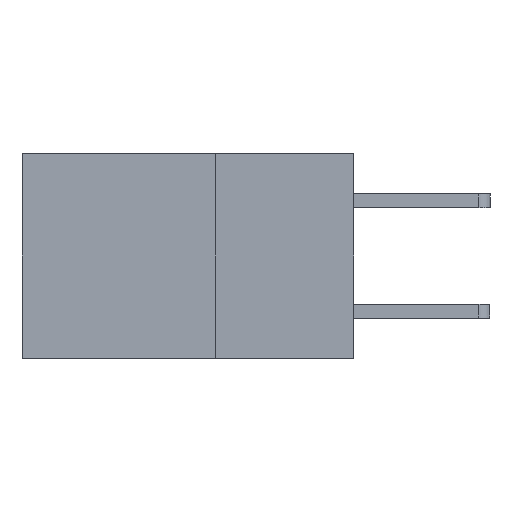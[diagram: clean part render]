
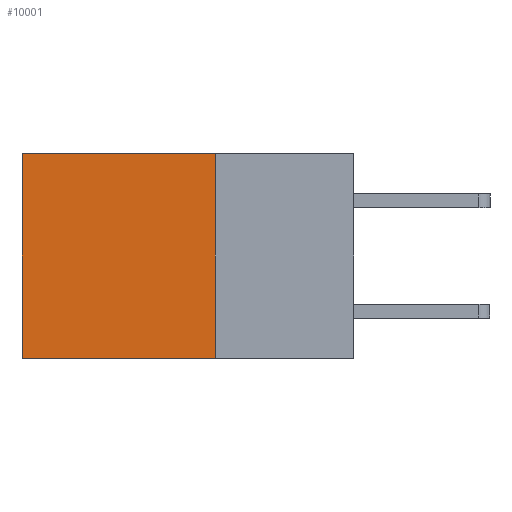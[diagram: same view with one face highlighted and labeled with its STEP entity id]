
A CAD part, left-side view. The second image highlights one B-rep face of the part: STEP entity #10001.
In plain terms, the highlighted planar face has unit normal (-1, 0, 0).
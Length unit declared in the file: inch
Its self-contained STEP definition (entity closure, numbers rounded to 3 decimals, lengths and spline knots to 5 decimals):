
#481 = CARTESIAN_POINT ( 'NONE',  ( 0.2875, 0.6, 0. ) ) ;
#626 = DIRECTION ( 'NONE',  ( 0., 0., -1. ) ) ;
#1221 = CARTESIAN_POINT ( 'NONE',  ( 0.2875, 0.25, 0. ) ) ;
#1279 = CARTESIAN_POINT ( 'NONE',  ( 0.2875, 0.25, 0. ) ) ;
#1508 = CARTESIAN_POINT ( 'NONE',  ( 0.2875, 0.6, -0.37 ) ) ;
#1657 = EDGE_CURVE ( 'NONE', #10789, #1830, #7637, .T. ) ;
#1830 = VERTEX_POINT ( 'NONE', #9324 ) ;
#2373 = EDGE_CURVE ( 'NONE', #10789, #7812, #5882, .T. ) ;
#2756 = EDGE_LOOP ( 'NONE', ( #9676, #6191, #10970, #8024 ) ) ;
#2924 = DIRECTION ( 'NONE',  ( 0., 0., -1. ) ) ;
#2990 = PLANE ( 'NONE',  #8286 ) ;
#3038 = DIRECTION ( 'NONE',  ( 1., 0., 0. ) ) ;
#3912 = VERTEX_POINT ( 'NONE', #1508 ) ;
#4685 = VECTOR ( 'NONE', #9892, 39.37008 ) ;
#5512 = DIRECTION ( 'NONE',  ( 0., 1., 0. ) ) ;
#5693 = DIRECTION ( 'NONE',  ( 0., 1., 0. ) ) ;
#5858 = CARTESIAN_POINT ( 'NONE',  ( 0.2875, 0.6, 0. ) ) ;
#5882 = LINE ( 'NONE', #1221, #7065 ) ;
#6191 = ORIENTED_EDGE ( 'NONE', *, *, #6640, .F. ) ;
#6640 = EDGE_CURVE ( 'NONE', #1830, #3912, #7420, .T. ) ;
#6700 = CARTESIAN_POINT ( 'NONE',  ( 0.2875, 0.25, 0. ) ) ;
#7065 = VECTOR ( 'NONE', #5693, 39.37008 ) ;
#7067 = CARTESIAN_POINT ( 'NONE',  ( 0.2875, 0.25, 0. ) ) ;
#7420 = LINE ( 'NONE', #7998, #7594 ) ;
#7594 = VECTOR ( 'NONE', #5512, 39.37008 ) ;
#7637 = LINE ( 'NONE', #7067, #9256 ) ;
#7812 = VERTEX_POINT ( 'NONE', #5858 ) ;
#7998 = CARTESIAN_POINT ( 'NONE',  ( 0.2875, 0.25, -0.37 ) ) ;
#8024 = ORIENTED_EDGE ( 'NONE', *, *, #2373, .T. ) ;
#8286 = AXIS2_PLACEMENT_3D ( 'NONE', #1279, #3038, #2924 ) ;
#8808 = LINE ( 'NONE', #481, #4685 ) ;
#9256 = VECTOR ( 'NONE', #626, 39.37008 ) ;
#9324 = CARTESIAN_POINT ( 'NONE',  ( 0.2875, 0.25, -0.37 ) ) ;
#9504 = FACE_OUTER_BOUND ( 'NONE', #2756, .T. ) ;
#9676 = ORIENTED_EDGE ( 'NONE', *, *, #11789, .T. ) ;
#9892 = DIRECTION ( 'NONE',  ( 0., 0., -1. ) ) ;
#10001 = ADVANCED_FACE ( 'NONE', ( #9504 ), #2990, .F. ) ;
#10789 = VERTEX_POINT ( 'NONE', #6700 ) ;
#10970 = ORIENTED_EDGE ( 'NONE', *, *, #1657, .F. ) ;
#11789 = EDGE_CURVE ( 'NONE', #7812, #3912, #8808, .T. ) ;
